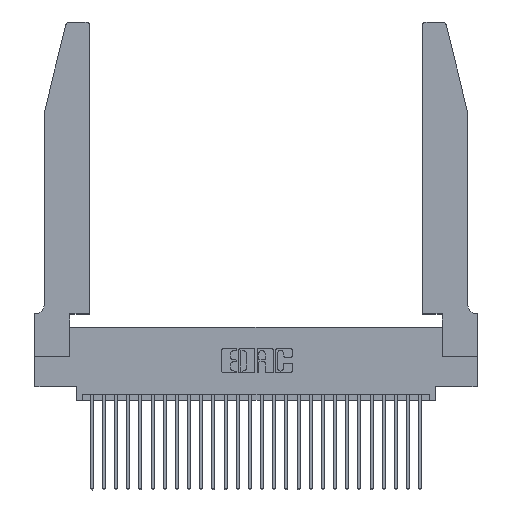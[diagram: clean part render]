
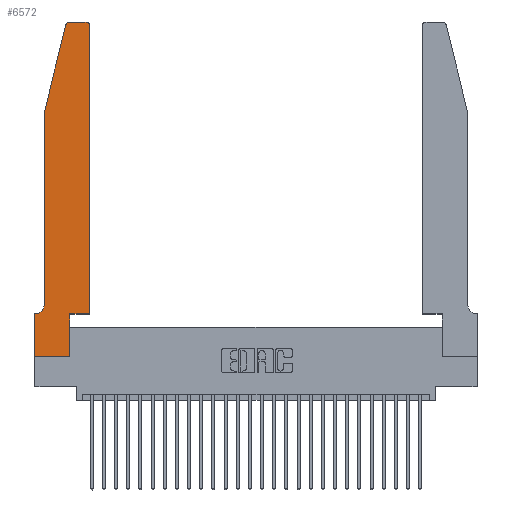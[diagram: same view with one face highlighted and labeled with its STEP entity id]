
A CAD part, top view. The second image highlights one B-rep face of the part: STEP entity #6572.
In plain terms, the highlighted planar face has unit normal (0, 0, 1).
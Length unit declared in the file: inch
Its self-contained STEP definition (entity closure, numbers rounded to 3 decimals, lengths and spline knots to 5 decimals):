
#221 = LINE ( 'NONE', #1283, #9967 ) ;
#471 = CARTESIAN_POINT ( 'NONE',  ( 0.4505, 0.35, 0.37 ) ) ;
#618 = CARTESIAN_POINT ( 'NONE',  ( 0.284, 2.75, 0.37 ) ) ;
#660 = CARTESIAN_POINT ( 'NONE',  ( 0.2865, 0., 0.37 ) ) ;
#727 = ORIENTED_EDGE ( 'NONE', *, *, #7469, .T. ) ;
#864 = CIRCLE ( 'NONE', #16024, 0.03 ) ;
#983 = VERTEX_POINT ( 'NONE', #2502 ) ;
#1034 = ORIENTED_EDGE ( 'NONE', *, *, #20691, .T. ) ;
#1180 = CARTESIAN_POINT ( 'NONE',  ( 0.4205, 2.75, 0.37 ) ) ;
#1200 = CARTESIAN_POINT ( 'NONE',  ( 0.284, 2.72, 0.37 ) ) ;
#1283 = CARTESIAN_POINT ( 'NONE',  ( 0.4505, 0.35, 0.37 ) ) ;
#2272 = ORIENTED_EDGE ( 'NONE', *, *, #3089, .T. ) ;
#2323 = AXIS2_PLACEMENT_3D ( 'NONE', #11017, #28682, #4207 ) ;
#2405 = DIRECTION ( 'NONE',  ( 0., 1., 0. ) ) ;
#2502 = CARTESIAN_POINT ( 'NONE',  ( 0.0755, 0.42, 0.37 ) ) ;
#2549 = DIRECTION ( 'NONE',  ( 0., -1., 0. ) ) ;
#3089 = EDGE_CURVE ( 'NONE', #16925, #9379, #5119, .T. ) ;
#3422 = DIRECTION ( 'NONE',  ( 1., 0., 0. ) ) ;
#3717 = VERTEX_POINT ( 'NONE', #25354 ) ;
#3854 = ORIENTED_EDGE ( 'NONE', *, *, #11879, .T. ) ;
#3942 = CIRCLE ( 'NONE', #13233, 0.07 ) ;
#3944 = CARTESIAN_POINT ( 'NONE',  ( 0.0755, 0.35, 0.37 ) ) ;
#4094 = CARTESIAN_POINT ( 'NONE',  ( 0.4505, 2.72, 0.37 ) ) ;
#4207 = DIRECTION ( 'NONE',  ( 1., 0., 0. ) ) ;
#4273 = LINE ( 'NONE', #18534, #15423 ) ;
#4281 = EDGE_CURVE ( 'NONE', #3717, #16914, #14449, .T. ) ;
#4865 = ORIENTED_EDGE ( 'NONE', *, *, #12512, .T. ) ;
#5119 = LINE ( 'NONE', #17163, #28404 ) ;
#5442 = CARTESIAN_POINT ( 'NONE',  ( 0.0755, 2., 0.37 ) ) ;
#5508 = VECTOR ( 'NONE', #2549, 39.37008 ) ;
#5715 = VERTEX_POINT ( 'NONE', #660 ) ;
#6572 = ADVANCED_FACE ( 'NONE', ( #23024 ), #15304, .T. ) ;
#6619 = DIRECTION ( 'NONE',  ( 1., 0., 0. ) ) ;
#7239 = LINE ( 'NONE', #8597, #5508 ) ;
#7335 = ORIENTED_EDGE ( 'NONE', *, *, #28725, .T. ) ;
#7469 = EDGE_CURVE ( 'NONE', #16914, #5715, #24421, .T. ) ;
#8597 = CARTESIAN_POINT ( 'NONE',  ( 0.0755, 2., 0.37 ) ) ;
#9041 = CARTESIAN_POINT ( 'NONE',  ( 0.2865, 0.35, 0.37 ) ) ;
#9121 = AXIS2_PLACEMENT_3D ( 'NONE', #14785, #16858, #3422 ) ;
#9379 = VERTEX_POINT ( 'NONE', #5442 ) ;
#9802 = VERTEX_POINT ( 'NONE', #14058 ) ;
#9967 = VECTOR ( 'NONE', #28189, 39.37008 ) ;
#10593 = EDGE_CURVE ( 'NONE', #17059, #16820, #221, .T. ) ;
#10602 = EDGE_CURVE ( 'NONE', #20721, #20390, #27356, .T. ) ;
#11017 = CARTESIAN_POINT ( 'NONE',  ( 0., 0.35, 0.37 ) ) ;
#11879 = EDGE_CURVE ( 'NONE', #5715, #17059, #22075, .T. ) ;
#11957 = CARTESIAN_POINT ( 'NONE',  ( 0., 0., 0.37 ) ) ;
#12153 = CARTESIAN_POINT ( 'NONE',  ( 0.2865, 0.35, 0.37 ) ) ;
#12490 = EDGE_CURVE ( 'NONE', #20390, #26067, #4273, .T. ) ;
#12512 = EDGE_CURVE ( 'NONE', #983, #9802, #3942, .T. ) ;
#12965 = ORIENTED_EDGE ( 'NONE', *, *, #22273, .T. ) ;
#13049 = VECTOR ( 'NONE', #20659, 39.37008 ) ;
#13233 = AXIS2_PLACEMENT_3D ( 'NONE', #24920, #22782, #25300 ) ;
#13407 = LINE ( 'NONE', #25199, #13049 ) ;
#13763 = DIRECTION ( 'NONE',  ( -1., 0., 0. ) ) ;
#14058 = CARTESIAN_POINT ( 'NONE',  ( 0.0055, 0.35, 0.37 ) ) ;
#14101 = VECTOR ( 'NONE', #26485, 39.37008 ) ;
#14449 = LINE ( 'NONE', #20022, #21745 ) ;
#14785 = CARTESIAN_POINT ( 'NONE',  ( 0.4205, 2.72, 0.37 ) ) ;
#15267 = CARTESIAN_POINT ( 'NONE',  ( 0., 0., 0.37 ) ) ;
#15304 = PLANE ( 'NONE',  #2323 ) ;
#15423 = VECTOR ( 'NONE', #13763, 39.37008 ) ;
#15989 = ORIENTED_EDGE ( 'NONE', *, *, #28433, .T. ) ;
#16024 = AXIS2_PLACEMENT_3D ( 'NONE', #1200, #27448, #18921 ) ;
#16082 = ORIENTED_EDGE ( 'NONE', *, *, #4281, .T. ) ;
#16820 = VERTEX_POINT ( 'NONE', #471 ) ;
#16858 = DIRECTION ( 'NONE',  ( 0., 0., 1. ) ) ;
#16914 = VERTEX_POINT ( 'NONE', #11957 ) ;
#16925 = VERTEX_POINT ( 'NONE', #25053 ) ;
#16973 = DIRECTION ( 'NONE',  ( -0.239, -0.971, 0. ) ) ;
#17059 = VERTEX_POINT ( 'NONE', #12153 ) ;
#17163 = CARTESIAN_POINT ( 'NONE',  ( 0.0755, 2., 0.37 ) ) ;
#17837 = VECTOR ( 'NONE', #6619, 39.37008 ) ;
#18534 = CARTESIAN_POINT ( 'NONE',  ( 0.2605, 2.75, 0.37 ) ) ;
#18921 = DIRECTION ( 'NONE',  ( 1., 0., 0. ) ) ;
#20008 = LINE ( 'NONE', #3944, #14101 ) ;
#20022 = CARTESIAN_POINT ( 'NONE',  ( 0., 0., 0.37 ) ) ;
#20123 = DIRECTION ( 'NONE',  ( 0., -1., 0. ) ) ;
#20390 = VERTEX_POINT ( 'NONE', #1180 ) ;
#20659 = DIRECTION ( 'NONE',  ( 0., 1., 0. ) ) ;
#20691 = EDGE_CURVE ( 'NONE', #9379, #983, #7239, .T. ) ;
#20721 = VERTEX_POINT ( 'NONE', #4094 ) ;
#21517 = ORIENTED_EDGE ( 'NONE', *, *, #10593, .T. ) ;
#21745 = VECTOR ( 'NONE', #20123, 39.37008 ) ;
#22075 = LINE ( 'NONE', #9041, #27285 ) ;
#22139 = EDGE_LOOP ( 'NONE', ( #22669, #12965, #2272, #1034, #4865, #15989, #16082, #727, #3854, #21517, #7335, #26162 ) ) ;
#22273 = EDGE_CURVE ( 'NONE', #26067, #16925, #864, .T. ) ;
#22669 = ORIENTED_EDGE ( 'NONE', *, *, #12490, .T. ) ;
#22782 = DIRECTION ( 'NONE',  ( 0., 0., -1. ) ) ;
#23024 = FACE_OUTER_BOUND ( 'NONE', #22139, .T. ) ;
#24421 = LINE ( 'NONE', #15267, #17837 ) ;
#24920 = CARTESIAN_POINT ( 'NONE',  ( 0.0055, 0.42, 0.37 ) ) ;
#25053 = CARTESIAN_POINT ( 'NONE',  ( 0.25487, 2.72718, 0.37 ) ) ;
#25199 = CARTESIAN_POINT ( 'NONE',  ( 0.4505, 0.35, 0.37 ) ) ;
#25300 = DIRECTION ( 'NONE',  ( -1., 0., 0. ) ) ;
#25354 = CARTESIAN_POINT ( 'NONE',  ( 0., 0.35, 0.37 ) ) ;
#26067 = VERTEX_POINT ( 'NONE', #618 ) ;
#26162 = ORIENTED_EDGE ( 'NONE', *, *, #10602, .T. ) ;
#26485 = DIRECTION ( 'NONE',  ( -1., 0., 0. ) ) ;
#27285 = VECTOR ( 'NONE', #2405, 39.37008 ) ;
#27356 = CIRCLE ( 'NONE', #9121, 0.03 ) ;
#27448 = DIRECTION ( 'NONE',  ( 0., 0., 1. ) ) ;
#28189 = DIRECTION ( 'NONE',  ( 1., 0., 0. ) ) ;
#28404 = VECTOR ( 'NONE', #16973, 39.37008 ) ;
#28433 = EDGE_CURVE ( 'NONE', #9802, #3717, #20008, .T. ) ;
#28682 = DIRECTION ( 'NONE',  ( 0., 0., 1. ) ) ;
#28725 = EDGE_CURVE ( 'NONE', #16820, #20721, #13407, .T. ) ;
